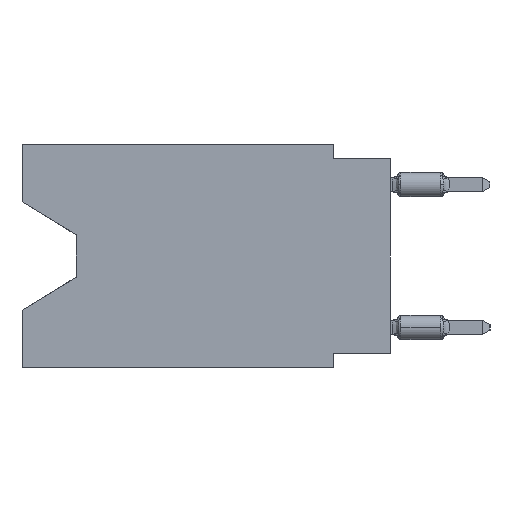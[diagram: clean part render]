
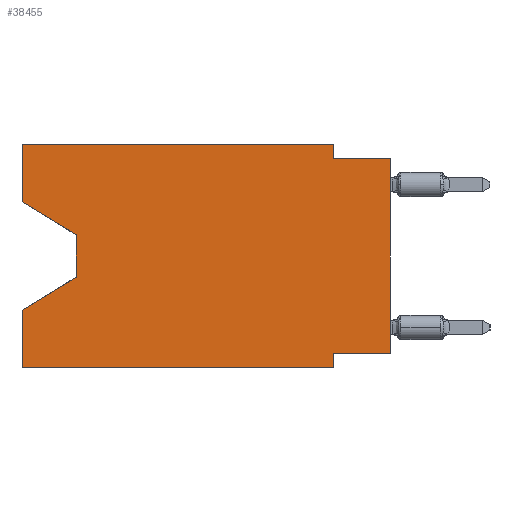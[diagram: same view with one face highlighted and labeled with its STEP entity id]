
A CAD part, left-side view. The second image highlights one B-rep face of the part: STEP entity #38455.
In plain terms, the highlighted planar face has unit normal (-1, 0, 0).
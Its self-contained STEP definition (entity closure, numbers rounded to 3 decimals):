
#301 = VECTOR ( 'NONE', #4924, 1000. ) ;
#448 = CARTESIAN_POINT ( 'NONE',  ( 0., 2.54, -9.906 ) ) ;
#1829 = LINE ( 'NONE', #2784, #10913 ) ;
#1946 = CARTESIAN_POINT ( 'NONE',  ( 0., 16.383, 0. ) ) ;
#1981 = ORIENTED_EDGE ( 'NONE', *, *, #40440, .F. ) ;
#2265 = VERTEX_POINT ( 'NONE', #6118 ) ;
#2784 = CARTESIAN_POINT ( 'NONE',  ( 0., 2.54, 0. ) ) ;
#4550 = CARTESIAN_POINT ( 'NONE',  ( 0., 2.54, -0.635 ) ) ;
#4651 = DIRECTION ( 'NONE',  ( 0., 0.855, -0.519 ) ) ;
#4884 = CARTESIAN_POINT ( 'NONE',  ( 0., 2.54, -9.271 ) ) ;
#4924 = DIRECTION ( 'NONE',  ( 0., 0., 1. ) ) ;
#6118 = CARTESIAN_POINT ( 'NONE',  ( 0., 16.383, -9.906 ) ) ;
#6154 = AXIS2_PLACEMENT_3D ( 'NONE', #28246, #21410, #18318 ) ;
#6528 = CARTESIAN_POINT ( 'NONE',  ( 0., 13.97, -4.013 ) ) ;
#6574 = VECTOR ( 'NONE', #39449, 1000. ) ;
#6657 = LINE ( 'NONE', #39035, #36247 ) ;
#6954 = DIRECTION ( 'NONE',  ( 0., 0., -1. ) ) ;
#7426 = EDGE_CURVE ( 'NONE', #36847, #24325, #13595, .T. ) ;
#7986 = CARTESIAN_POINT ( 'NONE',  ( 0., 13.97, -5.893 ) ) ;
#8255 = CARTESIAN_POINT ( 'NONE',  ( 0., 16.383, 0. ) ) ;
#8500 = EDGE_CURVE ( 'NONE', #20325, #21826, #31254, .T. ) ;
#8691 = ORIENTED_EDGE ( 'NONE', *, *, #11843, .F. ) ;
#8910 = CARTESIAN_POINT ( 'NONE',  ( 0., 16.383, -2.546 ) ) ;
#9070 = EDGE_LOOP ( 'NONE', ( #15078, #25647, #20341, #35991, #27515, #39706, #8691, #34132, #20695, #1981, #15088, #20443 ) ) ;
#9454 = LINE ( 'NONE', #40605, #22074 ) ;
#10071 = VECTOR ( 'NONE', #34708, 1000. ) ;
#10814 = LINE ( 'NONE', #30117, #6574 ) ;
#10913 = VECTOR ( 'NONE', #15842, 1000. ) ;
#11304 = VECTOR ( 'NONE', #4651, 1000. ) ;
#11843 = EDGE_CURVE ( 'NONE', #26935, #26939, #10814, .T. ) ;
#13595 = LINE ( 'NONE', #38906, #16053 ) ;
#14905 = VECTOR ( 'NONE', #20960, 1000. ) ;
#14985 = FACE_OUTER_BOUND ( 'NONE', #9070, .T. ) ;
#15078 = ORIENTED_EDGE ( 'NONE', *, *, #18245, .T. ) ;
#15088 = ORIENTED_EDGE ( 'NONE', *, *, #20918, .F. ) ;
#15842 = DIRECTION ( 'NONE',  ( 0., 0., -1. ) ) ;
#16053 = VECTOR ( 'NONE', #6954, 1000. ) ;
#16437 = DIRECTION ( 'NONE',  ( 0., 0., 1. ) ) ;
#16847 = LINE ( 'NONE', #448, #28838 ) ;
#17495 = EDGE_CURVE ( 'NONE', #26935, #19436, #38629, .T. ) ;
#17606 = CARTESIAN_POINT ( 'NONE',  ( 0., 2.54, -9.906 ) ) ;
#17657 = LINE ( 'NONE', #8910, #14905 ) ;
#18245 = EDGE_CURVE ( 'NONE', #20325, #36847, #17657, .T. ) ;
#18318 = DIRECTION ( 'NONE',  ( 0., 0., -1. ) ) ;
#18597 = DIRECTION ( 'NONE',  ( 0., 0., -1. ) ) ;
#19233 = CARTESIAN_POINT ( 'NONE',  ( 0., 0., -9.271 ) ) ;
#19436 = VERTEX_POINT ( 'NONE', #36173 ) ;
#19661 = VECTOR ( 'NONE', #28162, 1000. ) ;
#20170 = DIRECTION ( 'NONE',  ( 0., -1., 0. ) ) ;
#20325 = VERTEX_POINT ( 'NONE', #20875 ) ;
#20341 = ORIENTED_EDGE ( 'NONE', *, *, #23166, .T. ) ;
#20443 = ORIENTED_EDGE ( 'NONE', *, *, #8500, .F. ) ;
#20695 = ORIENTED_EDGE ( 'NONE', *, *, #38851, .F. ) ;
#20875 = CARTESIAN_POINT ( 'NONE',  ( 0., 16.383, -2.546 ) ) ;
#20918 = EDGE_CURVE ( 'NONE', #21826, #31093, #6657, .T. ) ;
#20960 = DIRECTION ( 'NONE',  ( 0., -0.855, -0.519 ) ) ;
#21410 = DIRECTION ( 'NONE',  ( 1., 0., 0. ) ) ;
#21826 = VERTEX_POINT ( 'NONE', #1946 ) ;
#22048 = CARTESIAN_POINT ( 'NONE',  ( 0., 16.383, -9.906 ) ) ;
#22074 = VECTOR ( 'NONE', #22319, 1000. ) ;
#22319 = DIRECTION ( 'NONE',  ( 0., -1., 0. ) ) ;
#23166 = EDGE_CURVE ( 'NONE', #24325, #30492, #32887, .T. ) ;
#23299 = CARTESIAN_POINT ( 'NONE',  ( 0., 0., 0. ) ) ;
#24024 = VERTEX_POINT ( 'NONE', #4550 ) ;
#24325 = VERTEX_POINT ( 'NONE', #25086 ) ;
#25086 = CARTESIAN_POINT ( 'NONE',  ( 0., 13.97, -5.893 ) ) ;
#25647 = ORIENTED_EDGE ( 'NONE', *, *, #7426, .T. ) ;
#25711 = VERTEX_POINT ( 'NONE', #17606 ) ;
#26864 = CARTESIAN_POINT ( 'NONE',  ( 0., 2.54, 0. ) ) ;
#26935 = VERTEX_POINT ( 'NONE', #19233 ) ;
#26939 = VERTEX_POINT ( 'NONE', #4884 ) ;
#27515 = ORIENTED_EDGE ( 'NONE', *, *, #36005, .T. ) ;
#28092 = LINE ( 'NONE', #22048, #10071 ) ;
#28162 = DIRECTION ( 'NONE',  ( 0., 0., 1. ) ) ;
#28246 = CARTESIAN_POINT ( 'NONE',  ( 0., 16.383, 0. ) ) ;
#28838 = VECTOR ( 'NONE', #18597, 1000. ) ;
#30117 = CARTESIAN_POINT ( 'NONE',  ( 0., 0., -9.271 ) ) ;
#30492 = VERTEX_POINT ( 'NONE', #34634 ) ;
#31093 = VERTEX_POINT ( 'NONE', #26864 ) ;
#31149 = PLANE ( 'NONE',  #6154 ) ;
#31254 = LINE ( 'NONE', #37692, #19661 ) ;
#31384 = VECTOR ( 'NONE', #16437, 1000. ) ;
#32574 = EDGE_CURVE ( 'NONE', #26939, #25711, #16847, .T. ) ;
#32887 = LINE ( 'NONE', #7986, #11304 ) ;
#34132 = ORIENTED_EDGE ( 'NONE', *, *, #17495, .T. ) ;
#34634 = CARTESIAN_POINT ( 'NONE',  ( 0., 16.383, -7.36 ) ) ;
#34708 = DIRECTION ( 'NONE',  ( 0., -1., 0. ) ) ;
#35991 = ORIENTED_EDGE ( 'NONE', *, *, #40416, .F. ) ;
#36005 = EDGE_CURVE ( 'NONE', #2265, #25711, #28092, .T. ) ;
#36173 = CARTESIAN_POINT ( 'NONE',  ( 0., 0., -0.635 ) ) ;
#36247 = VECTOR ( 'NONE', #20170, 1000. ) ;
#36689 = LINE ( 'NONE', #8255, #301 ) ;
#36847 = VERTEX_POINT ( 'NONE', #6528 ) ;
#37692 = CARTESIAN_POINT ( 'NONE',  ( 0., 16.383, 0. ) ) ;
#38455 = ADVANCED_FACE ( 'NONE', ( #14985 ), #31149, .F. ) ;
#38629 = LINE ( 'NONE', #23299, #31384 ) ;
#38851 = EDGE_CURVE ( 'NONE', #24024, #19436, #9454, .T. ) ;
#38906 = CARTESIAN_POINT ( 'NONE',  ( 0., 13.97, -4.013 ) ) ;
#39035 = CARTESIAN_POINT ( 'NONE',  ( 0., 16.383, 0. ) ) ;
#39449 = DIRECTION ( 'NONE',  ( 0., 1., 0. ) ) ;
#39706 = ORIENTED_EDGE ( 'NONE', *, *, #32574, .F. ) ;
#40416 = EDGE_CURVE ( 'NONE', #2265, #30492, #36689, .T. ) ;
#40440 = EDGE_CURVE ( 'NONE', #31093, #24024, #1829, .T. ) ;
#40605 = CARTESIAN_POINT ( 'NONE',  ( 0., 0., -0.635 ) ) ;
